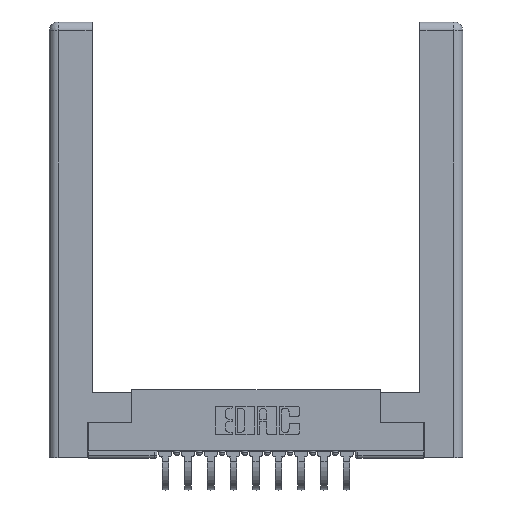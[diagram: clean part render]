
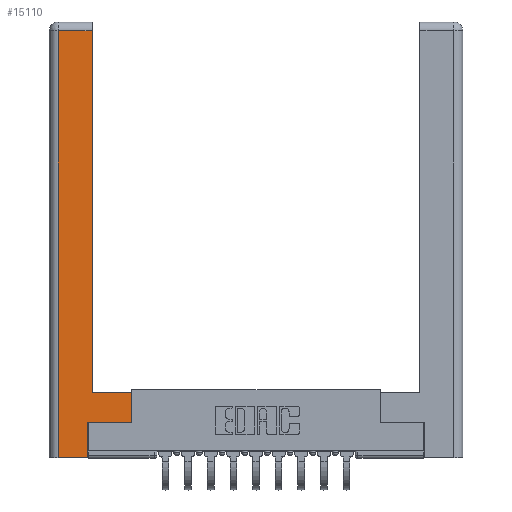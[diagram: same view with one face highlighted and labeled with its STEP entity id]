
A CAD part, top view. The second image highlights one B-rep face of the part: STEP entity #15110.
In plain terms, the highlighted planar face has unit normal (0, 0, 1).
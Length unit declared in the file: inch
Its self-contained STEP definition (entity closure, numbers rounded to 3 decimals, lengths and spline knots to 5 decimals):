
#287 = LINE ( 'NONE', #15428, #8153 ) ;
#413 = VECTOR ( 'NONE', #8355, 39.37008 ) ;
#419 = CARTESIAN_POINT ( 'NONE',  ( 0.295, 0.45, 0. ) ) ;
#757 = CARTESIAN_POINT ( 'NONE',  ( 0.565, 0.245, 0. ) ) ;
#829 = DIRECTION ( 'NONE',  ( 0., 1., 0. ) ) ;
#847 = LINE ( 'NONE', #1077, #14524 ) ;
#1077 = CARTESIAN_POINT ( 'NONE',  ( 0.0615, 0., 0. ) ) ;
#1775 = CARTESIAN_POINT ( 'NONE',  ( 0.0615, 2.94, 0. ) ) ;
#1835 = VERTEX_POINT ( 'NONE', #14756 ) ;
#1919 = VERTEX_POINT ( 'NONE', #11376 ) ;
#1947 = EDGE_CURVE ( 'NONE', #1835, #9291, #7538, .T. ) ;
#2708 = CARTESIAN_POINT ( 'NONE',  ( 0.265, 0., 0. ) ) ;
#3880 = VERTEX_POINT ( 'NONE', #11678 ) ;
#4015 = DIRECTION ( 'NONE',  ( 1., 0., 0. ) ) ;
#4255 = CARTESIAN_POINT ( 'NONE',  ( 0.295, 0.45, 0. ) ) ;
#4369 = EDGE_LOOP ( 'NONE', ( #4770, #13680, #9115, #12040, #5594, #16032, #9876, #8275 ) ) ;
#4770 = ORIENTED_EDGE ( 'NONE', *, *, #5411, .T. ) ;
#4964 = VECTOR ( 'NONE', #829, 39.37008 ) ;
#5411 = EDGE_CURVE ( 'NONE', #7521, #3880, #7038, .T. ) ;
#5594 = ORIENTED_EDGE ( 'NONE', *, *, #11984, .T. ) ;
#5951 = EDGE_CURVE ( 'NONE', #13146, #1835, #847, .T. ) ;
#5978 = EDGE_CURVE ( 'NONE', #3880, #13146, #9590, .T. ) ;
#6969 = LINE ( 'NONE', #757, #12380 ) ;
#7038 = LINE ( 'NONE', #10640, #4964 ) ;
#7236 = CARTESIAN_POINT ( 'NONE',  ( 0.265, 0.245, 0. ) ) ;
#7521 = VERTEX_POINT ( 'NONE', #4255 ) ;
#7538 = LINE ( 'NONE', #2708, #10502 ) ;
#7800 = VERTEX_POINT ( 'NONE', #15061 ) ;
#8153 = VECTOR ( 'NONE', #11406, 39.37008 ) ;
#8275 = ORIENTED_EDGE ( 'NONE', *, *, #12497, .T. ) ;
#8355 = DIRECTION ( 'NONE',  ( -1., 0., 0. ) ) ;
#8614 = DIRECTION ( 'NONE',  ( 0., 1., 0. ) ) ;
#9115 = ORIENTED_EDGE ( 'NONE', *, *, #5951, .T. ) ;
#9121 = PLANE ( 'NONE',  #9774 ) ;
#9291 = VERTEX_POINT ( 'NONE', #14233 ) ;
#9590 = LINE ( 'NONE', #14587, #413 ) ;
#9774 = AXIS2_PLACEMENT_3D ( 'NONE', #12886, #10423, #15437 ) ;
#9876 = ORIENTED_EDGE ( 'NONE', *, *, #10277, .T. ) ;
#10277 = EDGE_CURVE ( 'NONE', #1919, #15654, #287, .T. ) ;
#10423 = DIRECTION ( 'NONE',  ( 0., 0., -1. ) ) ;
#10502 = VECTOR ( 'NONE', #4015, 39.37008 ) ;
#10640 = CARTESIAN_POINT ( 'NONE',  ( 0.295, 3., 0. ) ) ;
#10795 = VECTOR ( 'NONE', #8614, 39.37008 ) ;
#10968 = DIRECTION ( 'NONE',  ( 0., -1., 0. ) ) ;
#11282 = DIRECTION ( 'NONE',  ( -1., 0., 0. ) ) ;
#11376 = CARTESIAN_POINT ( 'NONE',  ( 0.565, 0.245, 0. ) ) ;
#11406 = DIRECTION ( 'NONE',  ( 0., 1., 0. ) ) ;
#11413 = FACE_OUTER_BOUND ( 'NONE', #4369, .T. ) ;
#11678 = CARTESIAN_POINT ( 'NONE',  ( 0.295, 2.94, 0. ) ) ;
#11984 = EDGE_CURVE ( 'NONE', #9291, #7800, #13451, .T. ) ;
#12040 = ORIENTED_EDGE ( 'NONE', *, *, #1947, .T. ) ;
#12206 = EDGE_CURVE ( 'NONE', #7800, #1919, #6969, .T. ) ;
#12380 = VECTOR ( 'NONE', #15734, 39.37008 ) ;
#12497 = EDGE_CURVE ( 'NONE', #15654, #7521, #12674, .T. ) ;
#12674 = LINE ( 'NONE', #419, #15272 ) ;
#12886 = CARTESIAN_POINT ( 'NONE',  ( 0., 0., 0. ) ) ;
#13146 = VERTEX_POINT ( 'NONE', #1775 ) ;
#13451 = LINE ( 'NONE', #7236, #10795 ) ;
#13680 = ORIENTED_EDGE ( 'NONE', *, *, #5978, .T. ) ;
#14233 = CARTESIAN_POINT ( 'NONE',  ( 0.265, 0., 0. ) ) ;
#14524 = VECTOR ( 'NONE', #10968, 39.37008 ) ;
#14587 = CARTESIAN_POINT ( 'NONE',  ( 0.0615, 2.94, 0. ) ) ;
#14756 = CARTESIAN_POINT ( 'NONE',  ( 0.0615, 0., 0. ) ) ;
#15061 = CARTESIAN_POINT ( 'NONE',  ( 0.265, 0.245, 0. ) ) ;
#15110 = ADVANCED_FACE ( 'NONE', ( #11413 ), #9121, .F. ) ;
#15272 = VECTOR ( 'NONE', #11282, 39.37008 ) ;
#15428 = CARTESIAN_POINT ( 'NONE',  ( 0.565, 0.45, 0. ) ) ;
#15437 = DIRECTION ( 'NONE',  ( -1., 0., 0. ) ) ;
#15654 = VERTEX_POINT ( 'NONE', #15744 ) ;
#15734 = DIRECTION ( 'NONE',  ( 1., 0., 0. ) ) ;
#15744 = CARTESIAN_POINT ( 'NONE',  ( 0.565, 0.45, 0. ) ) ;
#16032 = ORIENTED_EDGE ( 'NONE', *, *, #12206, .T. ) ;
